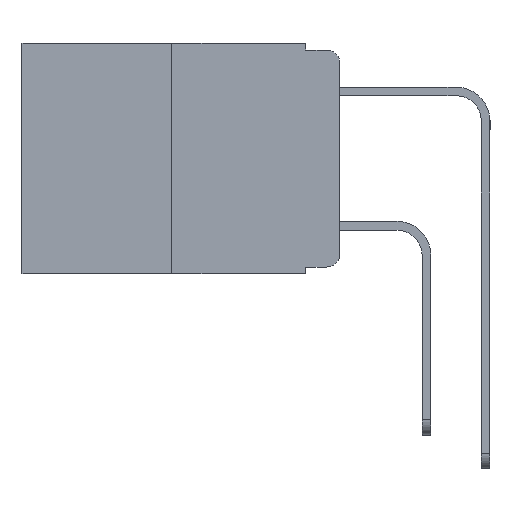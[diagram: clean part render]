
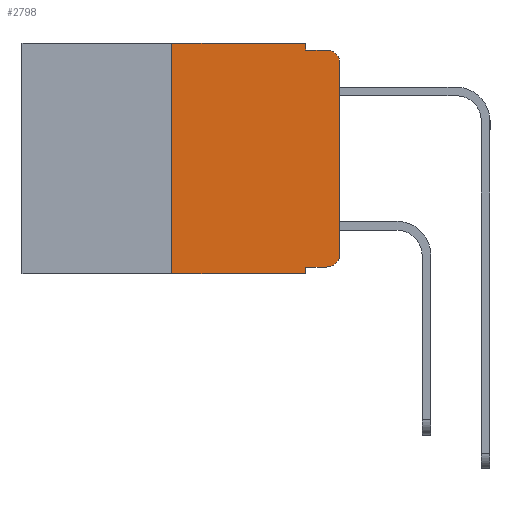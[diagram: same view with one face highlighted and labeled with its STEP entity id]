
A CAD part, left-side view. The second image highlights one B-rep face of the part: STEP entity #2798.
In plain terms, the highlighted planar face has unit normal (-1, 0, 0).
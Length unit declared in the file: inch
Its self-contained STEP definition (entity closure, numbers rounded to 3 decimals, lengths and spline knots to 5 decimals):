
#82 = DIRECTION ( 'NONE',  ( 0., -1., 0. ) ) ;
#333 = CARTESIAN_POINT ( 'NONE',  ( 0., 0.051, 0. ) ) ;
#353 = CARTESIAN_POINT ( 'NONE',  ( 0., 0.051, -0.01 ) ) ;
#492 = DIRECTION ( 'NONE',  ( 0., 0., -1. ) ) ;
#525 = DIRECTION ( 'NONE',  ( 1., 0., 0. ) ) ;
#691 = DIRECTION ( 'NONE',  ( 0., 0., -1. ) ) ;
#719 = DIRECTION ( 'NONE',  ( -1., 0., 0. ) ) ;
#792 = CARTESIAN_POINT ( 'NONE',  ( 0., 0.051, -0.343 ) ) ;
#793 = LINE ( 'NONE', #10701, #6083 ) ;
#988 = VERTEX_POINT ( 'NONE', #11088 ) ;
#1011 = CIRCLE ( 'NONE', #6514, 0.02 ) ;
#1030 = VECTOR ( 'NONE', #3155, 39.37008 ) ;
#1260 = CARTESIAN_POINT ( 'NONE',  ( 0., 0.051, -0.01 ) ) ;
#1319 = VERTEX_POINT ( 'NONE', #353 ) ;
#1393 = LINE ( 'NONE', #9594, #11529 ) ;
#1531 = VECTOR ( 'NONE', #8522, 39.37008 ) ;
#1539 = EDGE_CURVE ( 'NONE', #4330, #8074, #1011, .T. ) ;
#1823 = PLANE ( 'NONE',  #12026 ) ;
#1875 = LINE ( 'NONE', #333, #1531 ) ;
#2039 = CARTESIAN_POINT ( 'NONE',  ( 0., 0.473, 0. ) ) ;
#2565 = LINE ( 'NONE', #6423, #5067 ) ;
#2730 = CIRCLE ( 'NONE', #5647, 0.02 ) ;
#2798 = ADVANCED_FACE ( 'NONE', ( #10210 ), #1823, .F. ) ;
#2858 = ORIENTED_EDGE ( 'NONE', *, *, #11634, .T. ) ;
#3155 = DIRECTION ( 'NONE',  ( 0., -1., 0. ) ) ;
#3582 = LINE ( 'NONE', #5884, #5615 ) ;
#4175 = CARTESIAN_POINT ( 'NONE',  ( 0., 0.051, 0. ) ) ;
#4330 = VERTEX_POINT ( 'NONE', #6846 ) ;
#4366 = VECTOR ( 'NONE', #7960, 39.37008 ) ;
#4607 = ORIENTED_EDGE ( 'NONE', *, *, #1539, .T. ) ;
#4609 = CARTESIAN_POINT ( 'NONE',  ( 0., 0.02, -0.01 ) ) ;
#4754 = EDGE_LOOP ( 'NONE', ( #2858, #4607, #12597, #9177, #10480, #11468, #8126, #10511, #11792, #11058 ) ) ;
#5067 = VECTOR ( 'NONE', #82, 39.37008 ) ;
#5101 = VERTEX_POINT ( 'NONE', #9830 ) ;
#5615 = VECTOR ( 'NONE', #6824, 39.37008 ) ;
#5647 = AXIS2_PLACEMENT_3D ( 'NONE', #11642, #6056, #12572 ) ;
#5884 = CARTESIAN_POINT ( 'NONE',  ( 0., 0.051, -0.333 ) ) ;
#6010 = CARTESIAN_POINT ( 'NONE',  ( 0., 0.051, -0.333 ) ) ;
#6056 = DIRECTION ( 'NONE',  ( -1., 0., 0. ) ) ;
#6083 = VECTOR ( 'NONE', #11612, 39.37008 ) ;
#6423 = CARTESIAN_POINT ( 'NONE',  ( 0., 0.473, -0.343 ) ) ;
#6514 = AXIS2_PLACEMENT_3D ( 'NONE', #7325, #719, #691 ) ;
#6824 = DIRECTION ( 'NONE',  ( 0., -1., 0. ) ) ;
#6846 = CARTESIAN_POINT ( 'NONE',  ( 0., 0., -0.03 ) ) ;
#6878 = LINE ( 'NONE', #4175, #4366 ) ;
#7325 = CARTESIAN_POINT ( 'NONE',  ( 0., 0.02, -0.03 ) ) ;
#7897 = EDGE_CURVE ( 'NONE', #11907, #10985, #1875, .T. ) ;
#7929 = VERTEX_POINT ( 'NONE', #11320 ) ;
#7960 = DIRECTION ( 'NONE',  ( 0., 0., -1. ) ) ;
#8074 = VERTEX_POINT ( 'NONE', #4609 ) ;
#8126 = ORIENTED_EDGE ( 'NONE', *, *, #8929, .T. ) ;
#8522 = DIRECTION ( 'NONE',  ( 0., 0., -1. ) ) ;
#8531 = EDGE_CURVE ( 'NONE', #5101, #10609, #793, .T. ) ;
#8929 = EDGE_CURVE ( 'NONE', #5101, #10985, #2565, .T. ) ;
#9177 = ORIENTED_EDGE ( 'NONE', *, *, #11025, .F. ) ;
#9180 = EDGE_CURVE ( 'NONE', #12157, #988, #2730, .T. ) ;
#9423 = LINE ( 'NONE', #1260, #9741 ) ;
#9594 = CARTESIAN_POINT ( 'NONE',  ( 0., 0., 0. ) ) ;
#9741 = VECTOR ( 'NONE', #10204, 39.37008 ) ;
#9828 = EDGE_CURVE ( 'NONE', #11907, #12157, #3582, .T. ) ;
#9830 = CARTESIAN_POINT ( 'NONE',  ( 0., 0.25, -0.343 ) ) ;
#10204 = DIRECTION ( 'NONE',  ( 0., -1., 0. ) ) ;
#10210 = FACE_OUTER_BOUND ( 'NONE', #4754, .T. ) ;
#10424 = EDGE_CURVE ( 'NONE', #1319, #8074, #9423, .T. ) ;
#10480 = ORIENTED_EDGE ( 'NONE', *, *, #11109, .F. ) ;
#10493 = DIRECTION ( 'NONE',  ( 0., 0., 1. ) ) ;
#10511 = ORIENTED_EDGE ( 'NONE', *, *, #7897, .F. ) ;
#10609 = VERTEX_POINT ( 'NONE', #11261 ) ;
#10701 = CARTESIAN_POINT ( 'NONE',  ( 0., 0.25, 0. ) ) ;
#10985 = VERTEX_POINT ( 'NONE', #792 ) ;
#11025 = EDGE_CURVE ( 'NONE', #7929, #1319, #6878, .T. ) ;
#11058 = ORIENTED_EDGE ( 'NONE', *, *, #9180, .T. ) ;
#11088 = CARTESIAN_POINT ( 'NONE',  ( 0., 0., -0.313 ) ) ;
#11109 = EDGE_CURVE ( 'NONE', #10609, #7929, #11540, .T. ) ;
#11261 = CARTESIAN_POINT ( 'NONE',  ( 0., 0.25, 0. ) ) ;
#11320 = CARTESIAN_POINT ( 'NONE',  ( 0., 0.051, 0. ) ) ;
#11468 = ORIENTED_EDGE ( 'NONE', *, *, #8531, .F. ) ;
#11529 = VECTOR ( 'NONE', #10493, 39.37008 ) ;
#11540 = LINE ( 'NONE', #2039, #1030 ) ;
#11612 = DIRECTION ( 'NONE',  ( 0., 0., 1. ) ) ;
#11634 = EDGE_CURVE ( 'NONE', #988, #4330, #1393, .T. ) ;
#11642 = CARTESIAN_POINT ( 'NONE',  ( 0., 0.02, -0.313 ) ) ;
#11655 = CARTESIAN_POINT ( 'NONE',  ( 0., 0.473, 0. ) ) ;
#11792 = ORIENTED_EDGE ( 'NONE', *, *, #9828, .T. ) ;
#11907 = VERTEX_POINT ( 'NONE', #6010 ) ;
#12026 = AXIS2_PLACEMENT_3D ( 'NONE', #11655, #525, #492 ) ;
#12157 = VERTEX_POINT ( 'NONE', #12261 ) ;
#12261 = CARTESIAN_POINT ( 'NONE',  ( 0., 0.02, -0.333 ) ) ;
#12572 = DIRECTION ( 'NONE',  ( 0., 0., -1. ) ) ;
#12597 = ORIENTED_EDGE ( 'NONE', *, *, #10424, .F. ) ;
